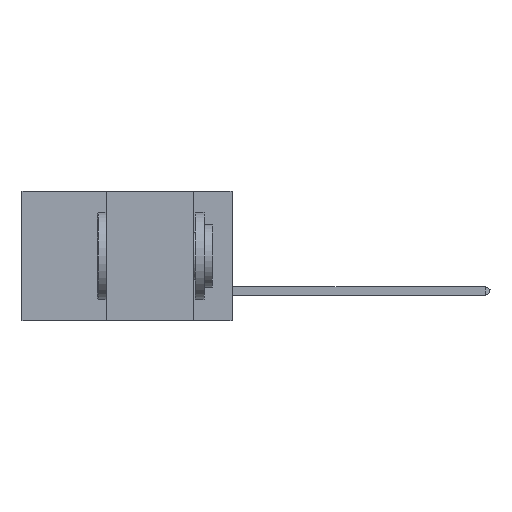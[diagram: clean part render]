
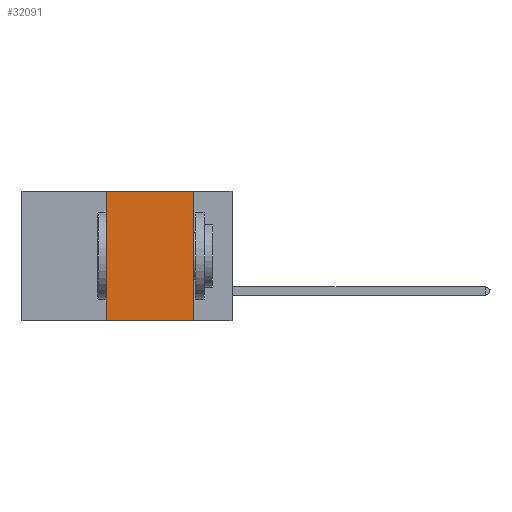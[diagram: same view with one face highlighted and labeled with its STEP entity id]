
A CAD part, left-side view. The second image highlights one B-rep face of the part: STEP entity #32091.
In plain terms, the highlighted planar face has unit normal (-1, 0, 0).
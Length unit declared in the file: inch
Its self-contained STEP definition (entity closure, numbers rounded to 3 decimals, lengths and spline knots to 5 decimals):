
#823 = LINE ( 'NONE', #28982, #33895 ) ;
#1448 = LINE ( 'NONE', #40957, #38159 ) ;
#3025 = CARTESIAN_POINT ( 'NONE',  ( 0., 0.6, 0. ) ) ;
#5973 = CARTESIAN_POINT ( 'NONE',  ( 0., 0.36, -0.37 ) ) ;
#6657 = DIRECTION ( 'NONE',  ( 0., 0., 1. ) ) ;
#9577 = DIRECTION ( 'NONE',  ( 0., -1., 0. ) ) ;
#9584 = EDGE_CURVE ( 'NONE', #17650, #27332, #25138, .T. ) ;
#11463 = ORIENTED_EDGE ( 'NONE', *, *, #28827, .T. ) ;
#11504 = CARTESIAN_POINT ( 'NONE',  ( 0., 0.11, 0. ) ) ;
#12391 = VECTOR ( 'NONE', #16075, 39.37008 ) ;
#12509 = CARTESIAN_POINT ( 'NONE',  ( 0., 0.11, -0.37 ) ) ;
#16075 = DIRECTION ( 'NONE',  ( 0., -1., 0. ) ) ;
#16091 = PLANE ( 'NONE',  #28005 ) ;
#17268 = ORIENTED_EDGE ( 'NONE', *, *, #38569, .F. ) ;
#17650 = VERTEX_POINT ( 'NONE', #17848 ) ;
#17848 = CARTESIAN_POINT ( 'NONE',  ( 0., 0.36, 0. ) ) ;
#18415 = EDGE_CURVE ( 'NONE', #27332, #38400, #23670, .T. ) ;
#21524 = ORIENTED_EDGE ( 'NONE', *, *, #18415, .F. ) ;
#23670 = LINE ( 'NONE', #31791, #42026 ) ;
#25138 = LINE ( 'NONE', #3025, #12391 ) ;
#25396 = DIRECTION ( 'NONE',  ( 1., 0., 0. ) ) ;
#27332 = VERTEX_POINT ( 'NONE', #11504 ) ;
#27741 = VERTEX_POINT ( 'NONE', #5973 ) ;
#28005 = AXIS2_PLACEMENT_3D ( 'NONE', #35289, #25396, #35434 ) ;
#28827 = EDGE_CURVE ( 'NONE', #27741, #38400, #823, .T. ) ;
#28982 = CARTESIAN_POINT ( 'NONE',  ( 0., 0.6, -0.37 ) ) ;
#29117 = FACE_OUTER_BOUND ( 'NONE', #31425, .T. ) ;
#31425 = EDGE_LOOP ( 'NONE', ( #21524, #34125, #17268, #11463 ) ) ;
#31791 = CARTESIAN_POINT ( 'NONE',  ( 0., 0.11, 0. ) ) ;
#32091 = ADVANCED_FACE ( 'NONE', ( #29117 ), #16091, .F. ) ;
#33895 = VECTOR ( 'NONE', #9577, 39.37008 ) ;
#34125 = ORIENTED_EDGE ( 'NONE', *, *, #9584, .F. ) ;
#35289 = CARTESIAN_POINT ( 'NONE',  ( 0., 0.6, 0. ) ) ;
#35434 = DIRECTION ( 'NONE',  ( 0., 0., -1. ) ) ;
#38159 = VECTOR ( 'NONE', #6657, 39.37008 ) ;
#38400 = VERTEX_POINT ( 'NONE', #12509 ) ;
#38569 = EDGE_CURVE ( 'NONE', #27741, #17650, #1448, .T. ) ;
#40957 = CARTESIAN_POINT ( 'NONE',  ( 0., 0.36, 0. ) ) ;
#41731 = DIRECTION ( 'NONE',  ( 0., 0., -1. ) ) ;
#42026 = VECTOR ( 'NONE', #41731, 39.37008 ) ;
